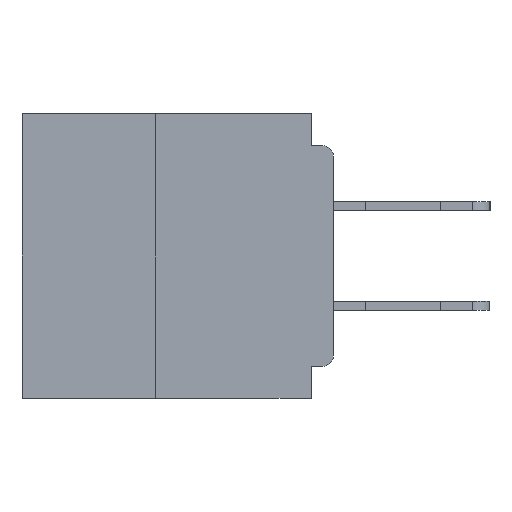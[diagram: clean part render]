
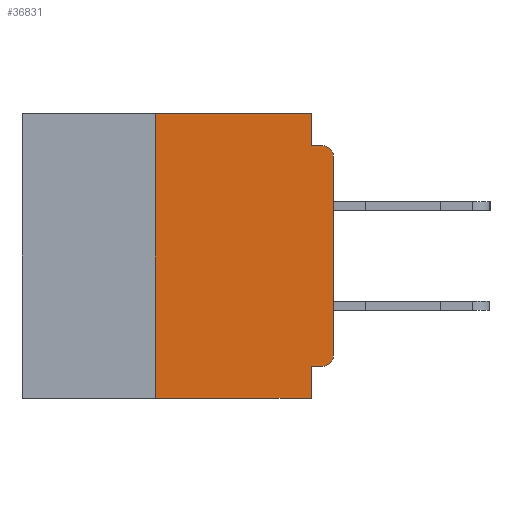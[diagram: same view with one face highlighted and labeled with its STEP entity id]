
A CAD part, left-side view. The second image highlights one B-rep face of the part: STEP entity #36831.
In plain terms, the highlighted planar face has unit normal (-1, 0, 0).
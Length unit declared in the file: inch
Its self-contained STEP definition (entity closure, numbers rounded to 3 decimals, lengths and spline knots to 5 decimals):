
#660 = CARTESIAN_POINT ( 'NONE',  ( 0., 0., -0.34 ) ) ;
#1287 = CARTESIAN_POINT ( 'NONE',  ( 0., 0.015, -0.045 ) ) ;
#2235 = VERTEX_POINT ( 'NONE', #30059 ) ;
#2237 = CARTESIAN_POINT ( 'NONE',  ( 0., 0., 0. ) ) ;
#3690 = ORIENTED_EDGE ( 'NONE', *, *, #9312, .F. ) ;
#4067 = VERTEX_POINT ( 'NONE', #15388 ) ;
#4593 = VERTEX_POINT ( 'NONE', #22915 ) ;
#4863 = CARTESIAN_POINT ( 'NONE',  ( 0., 0.25, -0.4 ) ) ;
#5936 = VECTOR ( 'NONE', #30394, 39.37008 ) ;
#5942 = CARTESIAN_POINT ( 'NONE',  ( 0., 0.437, 0. ) ) ;
#6072 = DIRECTION ( 'NONE',  ( 0., 0., -1. ) ) ;
#8128 = VECTOR ( 'NONE', #11168, 39.37008 ) ;
#8326 = AXIS2_PLACEMENT_3D ( 'NONE', #35800, #17213, #38948 ) ;
#8913 = VERTEX_POINT ( 'NONE', #15814 ) ;
#8986 = EDGE_CURVE ( 'NONE', #8913, #12086, #25744, .T. ) ;
#9241 = LINE ( 'NONE', #22082, #24871 ) ;
#9312 = EDGE_CURVE ( 'NONE', #12086, #20857, #22275, .T. ) ;
#9430 = VECTOR ( 'NONE', #10664, 39.37008 ) ;
#10664 = DIRECTION ( 'NONE',  ( 0., 0., -1. ) ) ;
#11168 = DIRECTION ( 'NONE',  ( 0., 0., 1. ) ) ;
#11405 = CARTESIAN_POINT ( 'NONE',  ( 0., 0., -0.045 ) ) ;
#11479 = ORIENTED_EDGE ( 'NONE', *, *, #21701, .T. ) ;
#12086 = VERTEX_POINT ( 'NONE', #32798 ) ;
#12976 = VECTOR ( 'NONE', #39307, 39.37008 ) ;
#13597 = CARTESIAN_POINT ( 'NONE',  ( 0., 0.437, 0. ) ) ;
#14000 = VECTOR ( 'NONE', #38745, 39.37008 ) ;
#14910 = CARTESIAN_POINT ( 'NONE',  ( 0., 0.015, -0.355 ) ) ;
#15388 = CARTESIAN_POINT ( 'NONE',  ( 0., 0., -0.06 ) ) ;
#15455 = FACE_OUTER_BOUND ( 'NONE', #32797, .T. ) ;
#15811 = DIRECTION ( 'NONE',  ( 0., -1., 0. ) ) ;
#15814 = CARTESIAN_POINT ( 'NONE',  ( 0., 0.031, 0. ) ) ;
#15964 = LINE ( 'NONE', #13597, #14000 ) ;
#16168 = CARTESIAN_POINT ( 'NONE',  ( 0., 0.031, -0.4 ) ) ;
#16424 = LINE ( 'NONE', #4863, #8128 ) ;
#16440 = VECTOR ( 'NONE', #22505, 39.37008 ) ;
#16494 = VERTEX_POINT ( 'NONE', #14910 ) ;
#16756 = LINE ( 'NONE', #38540, #9430 ) ;
#17213 = DIRECTION ( 'NONE',  ( -1., 0., 0. ) ) ;
#18105 = DIRECTION ( 'NONE',  ( -1., 0., 0. ) ) ;
#18278 = ORIENTED_EDGE ( 'NONE', *, *, #31850, .T. ) ;
#18509 = PLANE ( 'NONE',  #25695 ) ;
#20021 = VERTEX_POINT ( 'NONE', #16168 ) ;
#20500 = AXIS2_PLACEMENT_3D ( 'NONE', #36683, #18105, #39831 ) ;
#20857 = VERTEX_POINT ( 'NONE', #1287 ) ;
#21574 = LINE ( 'NONE', #2237, #5936 ) ;
#21701 = EDGE_CURVE ( 'NONE', #4067, #20857, #24144, .T. ) ;
#22082 = CARTESIAN_POINT ( 'NONE',  ( 0., 0.437, -0.4 ) ) ;
#22275 = LINE ( 'NONE', #11405, #12976 ) ;
#22386 = CIRCLE ( 'NONE', #8326, 0.015 ) ;
#22505 = DIRECTION ( 'NONE',  ( 0., 0., -1. ) ) ;
#22915 = CARTESIAN_POINT ( 'NONE',  ( 0., 0.25, -0.4 ) ) ;
#23438 = ORIENTED_EDGE ( 'NONE', *, *, #29967, .F. ) ;
#23641 = ORIENTED_EDGE ( 'NONE', *, *, #25236, .T. ) ;
#24144 = CIRCLE ( 'NONE', #20500, 0.015 ) ;
#24514 = ORIENTED_EDGE ( 'NONE', *, *, #8986, .F. ) ;
#24679 = CARTESIAN_POINT ( 'NONE',  ( 0., 0., -0.355 ) ) ;
#24792 = DIRECTION ( 'NONE',  ( 1., 0., 0. ) ) ;
#24871 = VECTOR ( 'NONE', #15811, 39.37008 ) ;
#25236 = EDGE_CURVE ( 'NONE', #16494, #30178, #22386, .T. ) ;
#25616 = EDGE_CURVE ( 'NONE', #4593, #20021, #9241, .T. ) ;
#25695 = AXIS2_PLACEMENT_3D ( 'NONE', #5942, #24792, #6072 ) ;
#25744 = LINE ( 'NONE', #34819, #16440 ) ;
#26081 = VECTOR ( 'NONE', #40266, 39.37008 ) ;
#29677 = ORIENTED_EDGE ( 'NONE', *, *, #36637, .F. ) ;
#29967 = EDGE_CURVE ( 'NONE', #16494, #35425, #34272, .T. ) ;
#30059 = CARTESIAN_POINT ( 'NONE',  ( 0., 0.25, 0. ) ) ;
#30178 = VERTEX_POINT ( 'NONE', #660 ) ;
#30394 = DIRECTION ( 'NONE',  ( 0., 0., 1. ) ) ;
#31125 = EDGE_CURVE ( 'NONE', #35425, #20021, #16756, .T. ) ;
#31850 = EDGE_CURVE ( 'NONE', #30178, #4067, #21574, .T. ) ;
#32797 = EDGE_LOOP ( 'NONE', ( #18278, #11479, #3690, #24514, #29677, #35195, #40252, #33359, #23438, #23641 ) ) ;
#32798 = CARTESIAN_POINT ( 'NONE',  ( 0., 0.031, -0.045 ) ) ;
#33359 = ORIENTED_EDGE ( 'NONE', *, *, #31125, .F. ) ;
#34272 = LINE ( 'NONE', #24679, #26081 ) ;
#34819 = CARTESIAN_POINT ( 'NONE',  ( 0., 0.031, 0. ) ) ;
#35195 = ORIENTED_EDGE ( 'NONE', *, *, #36121, .F. ) ;
#35425 = VERTEX_POINT ( 'NONE', #35684 ) ;
#35684 = CARTESIAN_POINT ( 'NONE',  ( 0., 0.031, -0.355 ) ) ;
#35800 = CARTESIAN_POINT ( 'NONE',  ( 0., 0.015, -0.34 ) ) ;
#36121 = EDGE_CURVE ( 'NONE', #4593, #2235, #16424, .T. ) ;
#36637 = EDGE_CURVE ( 'NONE', #2235, #8913, #15964, .T. ) ;
#36683 = CARTESIAN_POINT ( 'NONE',  ( 0., 0.015, -0.06 ) ) ;
#36831 = ADVANCED_FACE ( 'NONE', ( #15455 ), #18509, .F. ) ;
#38540 = CARTESIAN_POINT ( 'NONE',  ( 0., 0.031, -0.4 ) ) ;
#38745 = DIRECTION ( 'NONE',  ( 0., -1., 0. ) ) ;
#38948 = DIRECTION ( 'NONE',  ( 0., 0., -1. ) ) ;
#39307 = DIRECTION ( 'NONE',  ( 0., -1., 0. ) ) ;
#39831 = DIRECTION ( 'NONE',  ( 0., 0., -1. ) ) ;
#40252 = ORIENTED_EDGE ( 'NONE', *, *, #25616, .T. ) ;
#40266 = DIRECTION ( 'NONE',  ( 0., 1., 0. ) ) ;
